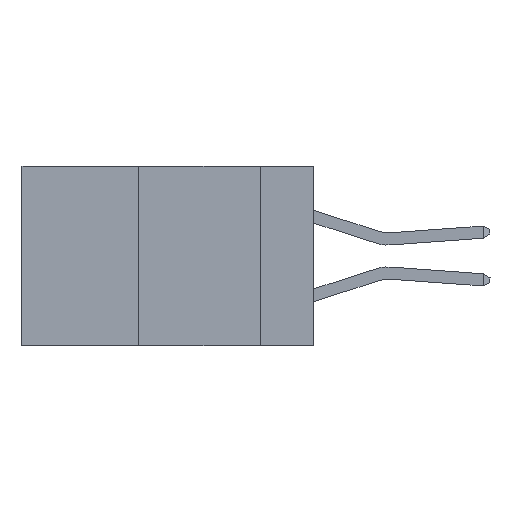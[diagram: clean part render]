
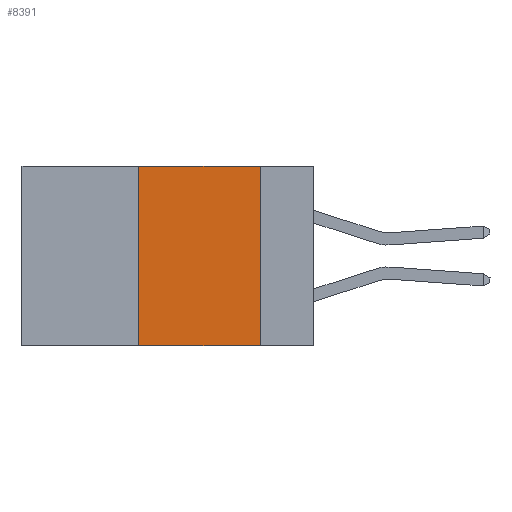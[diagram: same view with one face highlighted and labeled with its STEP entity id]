
A CAD part, left-side view. The second image highlights one B-rep face of the part: STEP entity #8391.
In plain terms, the highlighted planar face has unit normal (-1, 0, 0).
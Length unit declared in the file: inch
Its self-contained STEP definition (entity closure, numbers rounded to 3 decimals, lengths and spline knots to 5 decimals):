
#137 = FACE_OUTER_BOUND ( 'NONE', #28109, .T. ) ;
#780 = PLANE ( 'NONE',  #3198 ) ;
#2034 = VERTEX_POINT ( 'NONE', #23565 ) ;
#2719 = ORIENTED_EDGE ( 'NONE', *, *, #17051, .F. ) ;
#3198 = AXIS2_PLACEMENT_3D ( 'NONE', #12882, #28107, #22701 ) ;
#3878 = DIRECTION ( 'NONE',  ( 0., 0., 1. ) ) ;
#4247 = VERTEX_POINT ( 'NONE', #18589 ) ;
#6328 = CARTESIAN_POINT ( 'NONE',  ( 0., 0.36, 0. ) ) ;
#8391 = ADVANCED_FACE ( 'NONE', ( #137 ), #780, .F. ) ;
#8472 = DIRECTION ( 'NONE',  ( 0., -1., 0. ) ) ;
#8823 = DIRECTION ( 'NONE',  ( 0., 0., -1. ) ) ;
#9103 = LINE ( 'NONE', #6328, #26406 ) ;
#9322 = ORIENTED_EDGE ( 'NONE', *, *, #14234, .F. ) ;
#12110 = ORIENTED_EDGE ( 'NONE', *, *, #30606, .T. ) ;
#12882 = CARTESIAN_POINT ( 'NONE',  ( 0., 0.6, 0. ) ) ;
#12942 = VECTOR ( 'NONE', #8823, 39.37008 ) ;
#14234 = EDGE_CURVE ( 'NONE', #25015, #30750, #22971, .T. ) ;
#14955 = CARTESIAN_POINT ( 'NONE',  ( 0., 0.6, 0. ) ) ;
#17051 = EDGE_CURVE ( 'NONE', #2034, #25015, #9103, .T. ) ;
#18589 = CARTESIAN_POINT ( 'NONE',  ( 0., 0.11, -0.37 ) ) ;
#20013 = DIRECTION ( 'NONE',  ( 0., -1., 0. ) ) ;
#20084 = VECTOR ( 'NONE', #20013, 39.37008 ) ;
#20905 = CARTESIAN_POINT ( 'NONE',  ( 0., 0.6, -0.37 ) ) ;
#21244 = EDGE_CURVE ( 'NONE', #30750, #4247, #24040, .T. ) ;
#21266 = CARTESIAN_POINT ( 'NONE',  ( 0., 0.11, 0. ) ) ;
#22701 = DIRECTION ( 'NONE',  ( 0., 0., -1. ) ) ;
#22971 = LINE ( 'NONE', #14955, #20084 ) ;
#23523 = LINE ( 'NONE', #20905, #25334 ) ;
#23565 = CARTESIAN_POINT ( 'NONE',  ( 0., 0.36, -0.37 ) ) ;
#24040 = LINE ( 'NONE', #31257, #12942 ) ;
#24164 = ORIENTED_EDGE ( 'NONE', *, *, #21244, .F. ) ;
#25015 = VERTEX_POINT ( 'NONE', #27580 ) ;
#25334 = VECTOR ( 'NONE', #8472, 39.37008 ) ;
#26406 = VECTOR ( 'NONE', #3878, 39.37008 ) ;
#27580 = CARTESIAN_POINT ( 'NONE',  ( 0., 0.36, 0. ) ) ;
#28107 = DIRECTION ( 'NONE',  ( 1., 0., 0. ) ) ;
#28109 = EDGE_LOOP ( 'NONE', ( #24164, #9322, #2719, #12110 ) ) ;
#30606 = EDGE_CURVE ( 'NONE', #2034, #4247, #23523, .T. ) ;
#30750 = VERTEX_POINT ( 'NONE', #21266 ) ;
#31257 = CARTESIAN_POINT ( 'NONE',  ( 0., 0.11, 0. ) ) ;
